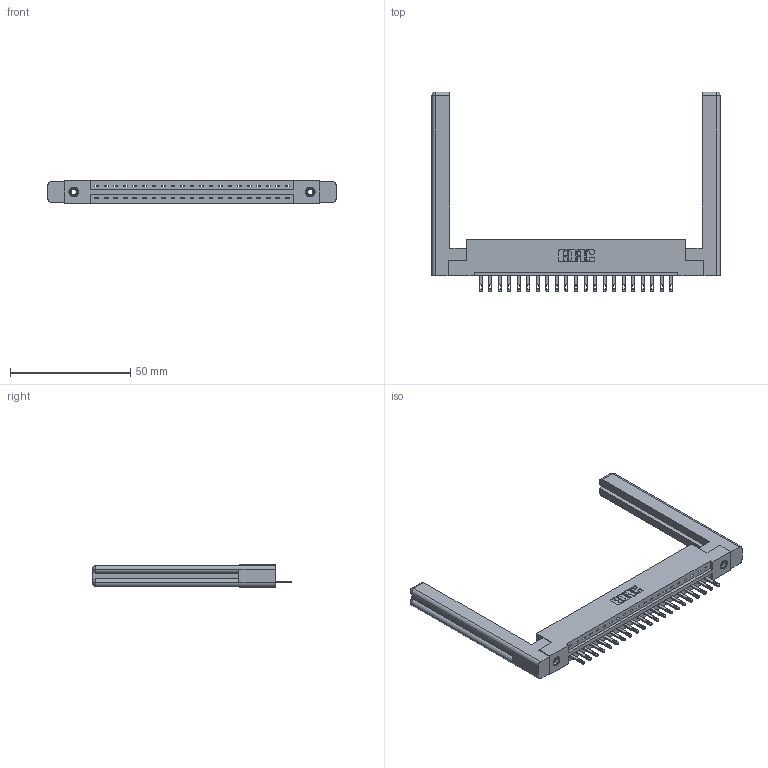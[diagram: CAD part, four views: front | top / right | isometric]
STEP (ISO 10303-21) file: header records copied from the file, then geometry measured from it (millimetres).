
FILE_DESCRIPTION (( 'STEP AP203' ), '1' );
FILE_NAME ('337-021-500-158.STEP', '2019-09-28T23:47:28', ( '' ), ( '' ), 'SwSTEP 2.0', 'SolidWorks 2016', '' );
FILE_SCHEMA (( 'CONFIG_CONTROL_DESIGN' ));
Length unit declared in the file: inch
Products named in the file (5): 345-250-001_345-250-001-102; 307-220-058; 337 Part_Flush Mounting Lugs - 0.156 Dia-TI; 345-292-001_345-293-100; 337-021-500-158
Assembly tree (26 placements, depth 2):
  337-021-500-158
    337 Part_Flush Mounting Lugs - 0.156 Dia-TI
    345-292-001_345-293-100  x21
    345-250-001_345-250-001-102  x2
    307-220-058  x2
Bounding box: 119.84 x 82.94 x 9.4 mm (x, y, z)
Volume: 19367.4 mm3; surface area: 17757.9 mm2
Topology: 26 solids, 26 shells, 1474 faces, 4445 edges, 2950 vertices
Faces by surface type: plane 994, cylinder 456, cone 12, torus 12
Entity records: 20890 total; most frequent: CARTESIAN_POINT 3636, ORIENTED_EDGE 3532, DIRECTION 3124, EDGE_CURVE 1766, LINE 1586, VECTOR 1586, VERTEX_POINT 1170, AXIS2_PLACEMENT_3D 769
